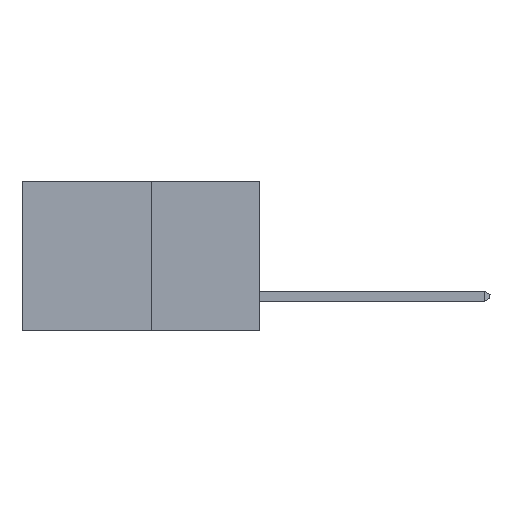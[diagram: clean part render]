
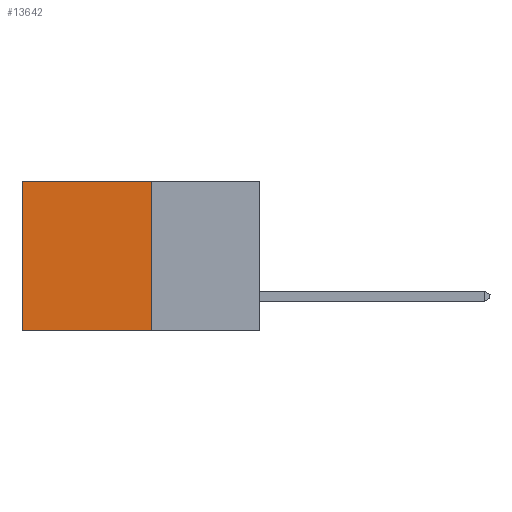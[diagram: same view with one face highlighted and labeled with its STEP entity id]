
A CAD part, left-side view. The second image highlights one B-rep face of the part: STEP entity #13642.
In plain terms, the highlighted planar face has unit normal (-1, 0, 0).
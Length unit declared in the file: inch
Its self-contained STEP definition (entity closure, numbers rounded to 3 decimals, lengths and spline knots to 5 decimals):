
#214 = LINE ( 'NONE', #798, #12080 ) ;
#798 = CARTESIAN_POINT ( 'NONE',  ( 0.277, 0.27, -0.37 ) ) ;
#845 = AXIS2_PLACEMENT_3D ( 'NONE', #7299, #2417, #10633 ) ;
#1118 = LINE ( 'NONE', #9633, #7155 ) ;
#1322 = CARTESIAN_POINT ( 'NONE',  ( 0.277, 0.27, -0.37 ) ) ;
#2417 = DIRECTION ( 'NONE',  ( 1., 0., 0. ) ) ;
#2690 = DIRECTION ( 'NONE',  ( 0., 1., 0. ) ) ;
#3030 = EDGE_CURVE ( 'NONE', #13704, #5810, #10531, .T. ) ;
#3156 = DIRECTION ( 'NONE',  ( 0., 0., -1. ) ) ;
#3998 = EDGE_CURVE ( 'NONE', #11973, #13704, #214, .T. ) ;
#4616 = DIRECTION ( 'NONE',  ( 0., 1., 0. ) ) ;
#5079 = FACE_OUTER_BOUND ( 'NONE', #11840, .T. ) ;
#5662 = ORIENTED_EDGE ( 'NONE', *, *, #3998, .F. ) ;
#5810 = VERTEX_POINT ( 'NONE', #7020 ) ;
#6210 = LINE ( 'NONE', #14473, #11755 ) ;
#6969 = EDGE_CURVE ( 'NONE', #11973, #7384, #6210, .T. ) ;
#6983 = ORIENTED_EDGE ( 'NONE', *, *, #7080, .T. ) ;
#7020 = CARTESIAN_POINT ( 'NONE',  ( 0.277, 0.59, -0.37 ) ) ;
#7073 = CARTESIAN_POINT ( 'NONE',  ( 0.277, 0.59, 0. ) ) ;
#7080 = EDGE_CURVE ( 'NONE', #7384, #5810, #1118, .T. ) ;
#7155 = VECTOR ( 'NONE', #10684, 39.37008 ) ;
#7299 = CARTESIAN_POINT ( 'NONE',  ( 0.277, 0.27, -0.37 ) ) ;
#7384 = VERTEX_POINT ( 'NONE', #7073 ) ;
#9594 = PLANE ( 'NONE',  #845 ) ;
#9633 = CARTESIAN_POINT ( 'NONE',  ( 0.277, 0.59, -0.37 ) ) ;
#9726 = CARTESIAN_POINT ( 'NONE',  ( 0.277, 0.27, -0.37 ) ) ;
#10104 = CARTESIAN_POINT ( 'NONE',  ( 0.277, 0.27, 0. ) ) ;
#10531 = LINE ( 'NONE', #9726, #12939 ) ;
#10633 = DIRECTION ( 'NONE',  ( 0., 0., -1. ) ) ;
#10684 = DIRECTION ( 'NONE',  ( 0., 0., -1. ) ) ;
#11755 = VECTOR ( 'NONE', #4616, 39.37008 ) ;
#11840 = EDGE_LOOP ( 'NONE', ( #6983, #13387, #5662, #12267 ) ) ;
#11973 = VERTEX_POINT ( 'NONE', #10104 ) ;
#12080 = VECTOR ( 'NONE', #3156, 39.37008 ) ;
#12267 = ORIENTED_EDGE ( 'NONE', *, *, #6969, .T. ) ;
#12939 = VECTOR ( 'NONE', #2690, 39.37008 ) ;
#13387 = ORIENTED_EDGE ( 'NONE', *, *, #3030, .F. ) ;
#13642 = ADVANCED_FACE ( 'NONE', ( #5079 ), #9594, .F. ) ;
#13704 = VERTEX_POINT ( 'NONE', #1322 ) ;
#14473 = CARTESIAN_POINT ( 'NONE',  ( 0.277, 0.27, 0. ) ) ;
